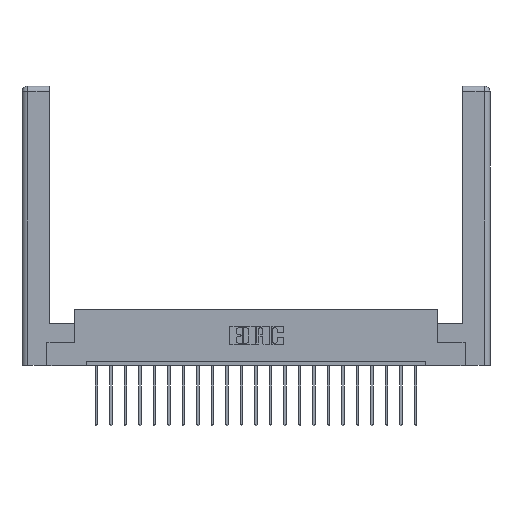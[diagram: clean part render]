
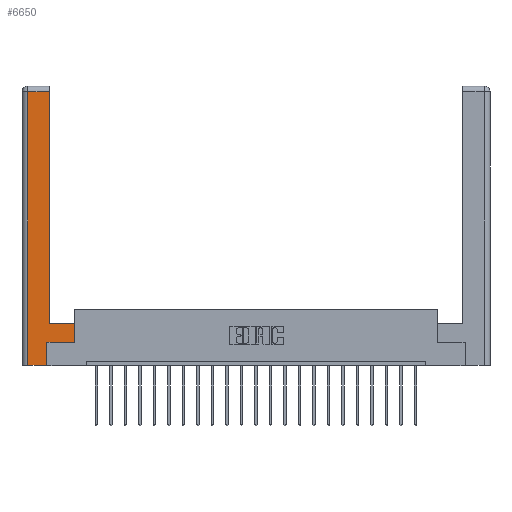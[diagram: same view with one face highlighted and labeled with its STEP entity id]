
A CAD part, top view. The second image highlights one B-rep face of the part: STEP entity #6650.
In plain terms, the highlighted planar face has unit normal (0, 0, 1).
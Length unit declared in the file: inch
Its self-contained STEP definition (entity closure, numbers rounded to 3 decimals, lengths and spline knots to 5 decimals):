
#227 = VERTEX_POINT ( 'NONE', #17668 ) ;
#351 = CARTESIAN_POINT ( 'NONE',  ( 0.0615, 0., 0. ) ) ;
#428 = ORIENTED_EDGE ( 'NONE', *, *, #2756, .T. ) ;
#1100 = CARTESIAN_POINT ( 'NONE',  ( 0.565, 0.45, 0. ) ) ;
#1381 = EDGE_CURVE ( 'NONE', #3049, #227, #11895, .T. ) ;
#2756 = EDGE_CURVE ( 'NONE', #6868, #14622, #10410, .T. ) ;
#3049 = VERTEX_POINT ( 'NONE', #8524 ) ;
#3309 = LINE ( 'NONE', #3438, #3846 ) ;
#3438 = CARTESIAN_POINT ( 'NONE',  ( 0.0615, 2.94, 0. ) ) ;
#3499 = VECTOR ( 'NONE', #12115, 39.37008 ) ;
#3694 = EDGE_LOOP ( 'NONE', ( #5518, #11148, #12003, #12113, #7651, #8581, #428, #5537 ) ) ;
#3846 = VECTOR ( 'NONE', #17126, 39.37008 ) ;
#4076 = VERTEX_POINT ( 'NONE', #20756 ) ;
#4403 = CARTESIAN_POINT ( 'NONE',  ( 0.295, 2.94, 0. ) ) ;
#4545 = LINE ( 'NONE', #21832, #4788 ) ;
#4788 = VECTOR ( 'NONE', #6619, 39.37008 ) ;
#5379 = DIRECTION ( 'NONE',  ( 1., 0., 0. ) ) ;
#5518 = ORIENTED_EDGE ( 'NONE', *, *, #12030, .T. ) ;
#5537 = ORIENTED_EDGE ( 'NONE', *, *, #9730, .T. ) ;
#6243 = DIRECTION ( 'NONE',  ( 0., 1., 0. ) ) ;
#6590 = EDGE_CURVE ( 'NONE', #18324, #4076, #3309, .T. ) ;
#6619 = DIRECTION ( 'NONE',  ( 0., 1., 0. ) ) ;
#6650 = ADVANCED_FACE ( 'NONE', ( #19644 ), #12377, .F. ) ;
#6868 = VERTEX_POINT ( 'NONE', #16894 ) ;
#7033 = VECTOR ( 'NONE', #6243, 39.37008 ) ;
#7395 = DIRECTION ( 'NONE',  ( -1., 0., 0. ) ) ;
#7651 = ORIENTED_EDGE ( 'NONE', *, *, #10499, .T. ) ;
#8287 = EDGE_CURVE ( 'NONE', #4076, #3049, #9673, .T. ) ;
#8471 = CARTESIAN_POINT ( 'NONE',  ( 0.265, 0., 0. ) ) ;
#8524 = CARTESIAN_POINT ( 'NONE',  ( 0.0615, 0., 0. ) ) ;
#8581 = ORIENTED_EDGE ( 'NONE', *, *, #12197, .T. ) ;
#9004 = CARTESIAN_POINT ( 'NONE',  ( 0.295, 0.45, 0. ) ) ;
#9340 = VECTOR ( 'NONE', #19964, 39.37008 ) ;
#9673 = LINE ( 'NONE', #351, #3499 ) ;
#9730 = EDGE_CURVE ( 'NONE', #14622, #13765, #18106, .T. ) ;
#10176 = VECTOR ( 'NONE', #14281, 39.37008 ) ;
#10410 = LINE ( 'NONE', #1100, #9340 ) ;
#10499 = EDGE_CURVE ( 'NONE', #227, #16338, #16382, .T. ) ;
#11140 = CARTESIAN_POINT ( 'NONE',  ( 0.565, 0.45, 0. ) ) ;
#11148 = ORIENTED_EDGE ( 'NONE', *, *, #6590, .T. ) ;
#11290 = CARTESIAN_POINT ( 'NONE',  ( 0.265, 0.245, 0. ) ) ;
#11895 = LINE ( 'NONE', #8471, #19708 ) ;
#12003 = ORIENTED_EDGE ( 'NONE', *, *, #8287, .T. ) ;
#12030 = EDGE_CURVE ( 'NONE', #13765, #18324, #4545, .T. ) ;
#12113 = ORIENTED_EDGE ( 'NONE', *, *, #1381, .T. ) ;
#12115 = DIRECTION ( 'NONE',  ( 0., -1., 0. ) ) ;
#12197 = EDGE_CURVE ( 'NONE', #16338, #6868, #20615, .T. ) ;
#12377 = PLANE ( 'NONE',  #18010 ) ;
#13765 = VERTEX_POINT ( 'NONE', #9004 ) ;
#13994 = DIRECTION ( 'NONE',  ( 0., 0., -1. ) ) ;
#14241 = CARTESIAN_POINT ( 'NONE',  ( 0., 0., 0. ) ) ;
#14281 = DIRECTION ( 'NONE',  ( 1., 0., 0. ) ) ;
#14622 = VERTEX_POINT ( 'NONE', #11140 ) ;
#15750 = VECTOR ( 'NONE', #16027, 39.37008 ) ;
#16027 = DIRECTION ( 'NONE',  ( -1., 0., 0. ) ) ;
#16338 = VERTEX_POINT ( 'NONE', #17194 ) ;
#16382 = LINE ( 'NONE', #11290, #7033 ) ;
#16894 = CARTESIAN_POINT ( 'NONE',  ( 0.565, 0.245, 0. ) ) ;
#17126 = DIRECTION ( 'NONE',  ( -1., 0., 0. ) ) ;
#17194 = CARTESIAN_POINT ( 'NONE',  ( 0.265, 0.245, 0. ) ) ;
#17668 = CARTESIAN_POINT ( 'NONE',  ( 0.265, 0., 0. ) ) ;
#18010 = AXIS2_PLACEMENT_3D ( 'NONE', #14241, #13994, #7395 ) ;
#18106 = LINE ( 'NONE', #19630, #15750 ) ;
#18324 = VERTEX_POINT ( 'NONE', #4403 ) ;
#19176 = CARTESIAN_POINT ( 'NONE',  ( 0.565, 0.245, 0. ) ) ;
#19630 = CARTESIAN_POINT ( 'NONE',  ( 0.295, 0.45, 0. ) ) ;
#19644 = FACE_OUTER_BOUND ( 'NONE', #3694, .T. ) ;
#19708 = VECTOR ( 'NONE', #5379, 39.37008 ) ;
#19964 = DIRECTION ( 'NONE',  ( 0., 1., 0. ) ) ;
#20615 = LINE ( 'NONE', #19176, #10176 ) ;
#20756 = CARTESIAN_POINT ( 'NONE',  ( 0.0615, 2.94, 0. ) ) ;
#21832 = CARTESIAN_POINT ( 'NONE',  ( 0.295, 3., 0. ) ) ;
